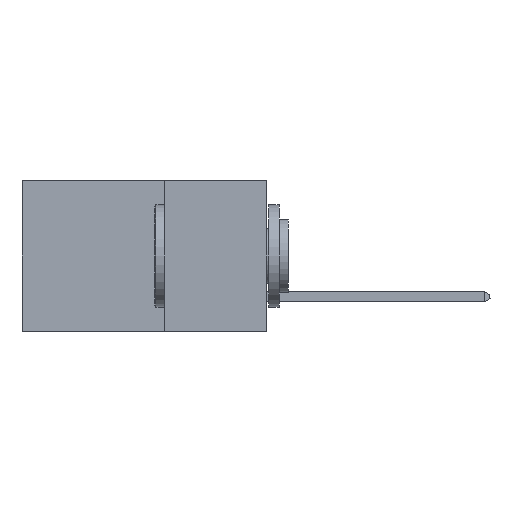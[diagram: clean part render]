
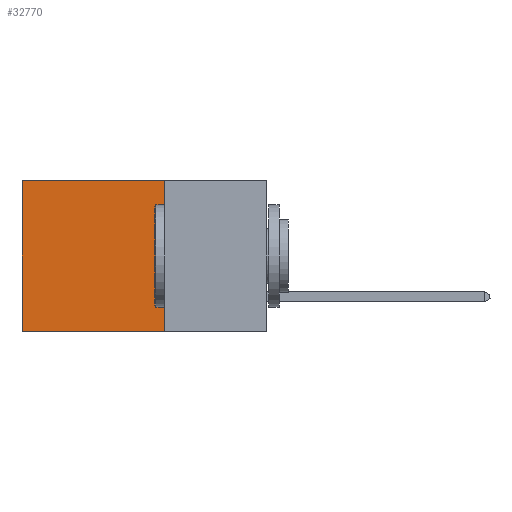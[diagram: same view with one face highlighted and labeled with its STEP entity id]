
A CAD part, left-side view. The second image highlights one B-rep face of the part: STEP entity #32770.
In plain terms, the highlighted planar face has unit normal (-1, 0, 0).
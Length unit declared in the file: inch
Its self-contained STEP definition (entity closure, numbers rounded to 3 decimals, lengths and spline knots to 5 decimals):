
#1044 = CARTESIAN_POINT ( 'NONE',  ( 0.2875, 0.25, 0. ) ) ;
#1812 = ORIENTED_EDGE ( 'NONE', *, *, #8981, .F. ) ;
#2044 = CARTESIAN_POINT ( 'NONE',  ( 0.2875, 0.6, 0. ) ) ;
#3588 = EDGE_CURVE ( 'NONE', #18129, #23994, #23259, .T. ) ;
#4204 = VERTEX_POINT ( 'NONE', #2044 ) ;
#6372 = VECTOR ( 'NONE', #9811, 39.37008 ) ;
#6712 = LINE ( 'NONE', #24415, #33528 ) ;
#8219 = CARTESIAN_POINT ( 'NONE',  ( 0.2875, 0.6, 0. ) ) ;
#8275 = DIRECTION ( 'NONE',  ( 0., 1., 0. ) ) ;
#8939 = DIRECTION ( 'NONE',  ( 1., 0., 0. ) ) ;
#8981 = EDGE_CURVE ( 'NONE', #23994, #9225, #6712, .T. ) ;
#9225 = VERTEX_POINT ( 'NONE', #22183 ) ;
#9772 = AXIS2_PLACEMENT_3D ( 'NONE', #19577, #8939, #17033 ) ;
#9811 = DIRECTION ( 'NONE',  ( 0., 1., 0. ) ) ;
#10035 = CARTESIAN_POINT ( 'NONE',  ( 0.2875, 0.25, -0.37 ) ) ;
#11264 = CARTESIAN_POINT ( 'NONE',  ( 0.2875, 0.25, 0. ) ) ;
#11472 = VECTOR ( 'NONE', #23972, 39.37008 ) ;
#11905 = LINE ( 'NONE', #8219, #11472 ) ;
#12074 = PLANE ( 'NONE',  #9772 ) ;
#15871 = LINE ( 'NONE', #23188, #6372 ) ;
#16970 = EDGE_LOOP ( 'NONE', ( #32329, #1812, #30958, #21199 ) ) ;
#17033 = DIRECTION ( 'NONE',  ( 0., 0., -1. ) ) ;
#18129 = VERTEX_POINT ( 'NONE', #11264 ) ;
#19577 = CARTESIAN_POINT ( 'NONE',  ( 0.2875, 0.25, 0. ) ) ;
#20352 = EDGE_CURVE ( 'NONE', #4204, #9225, #11905, .T. ) ;
#21199 = ORIENTED_EDGE ( 'NONE', *, *, #33059, .T. ) ;
#22183 = CARTESIAN_POINT ( 'NONE',  ( 0.2875, 0.6, -0.37 ) ) ;
#23188 = CARTESIAN_POINT ( 'NONE',  ( 0.2875, 0.25, 0. ) ) ;
#23259 = LINE ( 'NONE', #1044, #29008 ) ;
#23972 = DIRECTION ( 'NONE',  ( 0., 0., -1. ) ) ;
#23994 = VERTEX_POINT ( 'NONE', #10035 ) ;
#24415 = CARTESIAN_POINT ( 'NONE',  ( 0.2875, 0.25, -0.37 ) ) ;
#25792 = FACE_OUTER_BOUND ( 'NONE', #16970, .T. ) ;
#29008 = VECTOR ( 'NONE', #29780, 39.37008 ) ;
#29780 = DIRECTION ( 'NONE',  ( 0., 0., -1. ) ) ;
#30958 = ORIENTED_EDGE ( 'NONE', *, *, #3588, .F. ) ;
#32329 = ORIENTED_EDGE ( 'NONE', *, *, #20352, .T. ) ;
#32770 = ADVANCED_FACE ( 'NONE', ( #25792 ), #12074, .F. ) ;
#33059 = EDGE_CURVE ( 'NONE', #18129, #4204, #15871, .T. ) ;
#33528 = VECTOR ( 'NONE', #8275, 39.37008 ) ;
